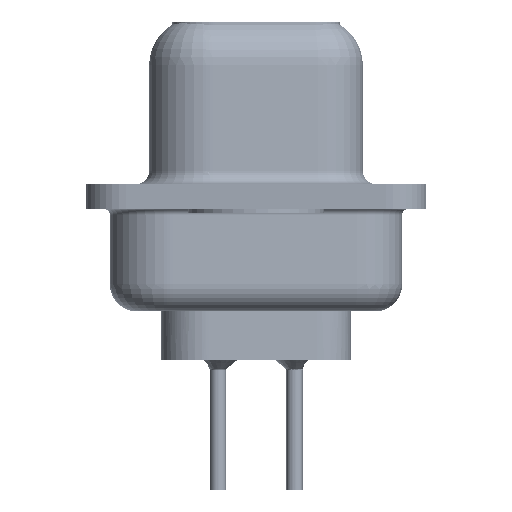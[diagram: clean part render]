
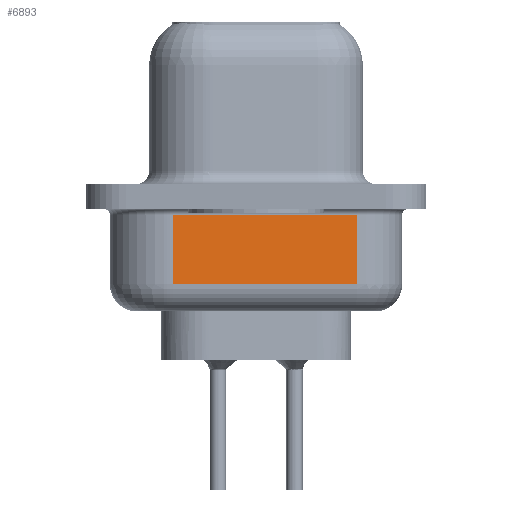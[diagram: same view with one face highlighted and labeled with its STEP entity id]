
A CAD part, left-side view. The second image highlights one B-rep face of the part: STEP entity #6893.
In plain terms, the highlighted planar face has unit normal (-0.985, -0.174, 0).
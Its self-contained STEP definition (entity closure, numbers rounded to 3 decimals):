
#304 = ORIENTED_EDGE ( 'NONE', *, *, #3986, .T. ) ;
#1300 = CARTESIAN_POINT ( 'NONE',  ( 2.88, 3.053, -4.25 ) ) ;
#1634 = VERTEX_POINT ( 'NONE', #14229 ) ;
#2130 = CARTESIAN_POINT ( 'NONE',  ( 4.079, -3.747, -0.7 ) ) ;
#2967 = DIRECTION ( 'NONE',  ( 0.174, -0.985, 0. ) ) ;
#3986 = EDGE_CURVE ( 'NONE', #13539, #18801, #4092, .T. ) ;
#4092 = LINE ( 'NONE', #14236, #23198 ) ;
#4177 = VECTOR ( 'NONE', #2967, 1000. ) ;
#4183 = EDGE_CURVE ( 'NONE', #1634, #9691, #14994, .T. ) ;
#4853 = DIRECTION ( 'NONE',  ( 0., 0., 1. ) ) ;
#5050 = CARTESIAN_POINT ( 'NONE',  ( 2.88, 3.053, -0.7 ) ) ;
#5799 = ORIENTED_EDGE ( 'NONE', *, *, #30003, .T. ) ;
#6893 = ADVANCED_FACE ( 'NONE', ( #17906 ), #20698, .F. ) ;
#9691 = VERTEX_POINT ( 'NONE', #10410 ) ;
#10298 = CARTESIAN_POINT ( 'NONE',  ( 2.88, 3.053, -4.25 ) ) ;
#10410 = CARTESIAN_POINT ( 'NONE',  ( 2.88, 3.053, -0.7 ) ) ;
#11771 = LINE ( 'NONE', #5050, #27995 ) ;
#12358 = CARTESIAN_POINT ( 'NONE',  ( 2.88, 3.053, -3.25 ) ) ;
#13539 = VERTEX_POINT ( 'NONE', #29576 ) ;
#14229 = CARTESIAN_POINT ( 'NONE',  ( 2.88, 3.053, -3.25 ) ) ;
#14236 = CARTESIAN_POINT ( 'NONE',  ( 4.079, -3.747, -4.25 ) ) ;
#14278 = DIRECTION ( 'NONE',  ( -0.174, 0.985, 0. ) ) ;
#14994 = LINE ( 'NONE', #10298, #22716 ) ;
#16210 = EDGE_LOOP ( 'NONE', ( #27363, #5799, #304, #19737 ) ) ;
#17906 = FACE_OUTER_BOUND ( 'NONE', #16210, .T. ) ;
#18801 = VERTEX_POINT ( 'NONE', #2130 ) ;
#19737 = ORIENTED_EDGE ( 'NONE', *, *, #25728, .T. ) ;
#20698 = PLANE ( 'NONE',  #25398 ) ;
#22356 = LINE ( 'NONE', #12358, #4177 ) ;
#22716 = VECTOR ( 'NONE', #4853, 1000. ) ;
#22745 = DIRECTION ( 'NONE',  ( 0.985, 0.174, 0. ) ) ;
#23198 = VECTOR ( 'NONE', #30555, 1000. ) ;
#25398 = AXIS2_PLACEMENT_3D ( 'NONE', #1300, #22745, #30294 ) ;
#25728 = EDGE_CURVE ( 'NONE', #18801, #9691, #11771, .T. ) ;
#27363 = ORIENTED_EDGE ( 'NONE', *, *, #4183, .F. ) ;
#27995 = VECTOR ( 'NONE', #14278, 1000. ) ;
#29576 = CARTESIAN_POINT ( 'NONE',  ( 4.079, -3.747, -3.25 ) ) ;
#30003 = EDGE_CURVE ( 'NONE', #1634, #13539, #22356, .T. ) ;
#30294 = DIRECTION ( 'NONE',  ( -0.174, 0.985, 0. ) ) ;
#30555 = DIRECTION ( 'NONE',  ( 0., 0., 1. ) ) ;
